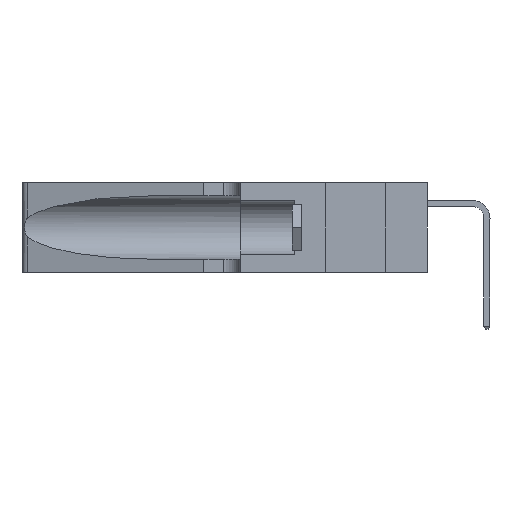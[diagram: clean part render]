
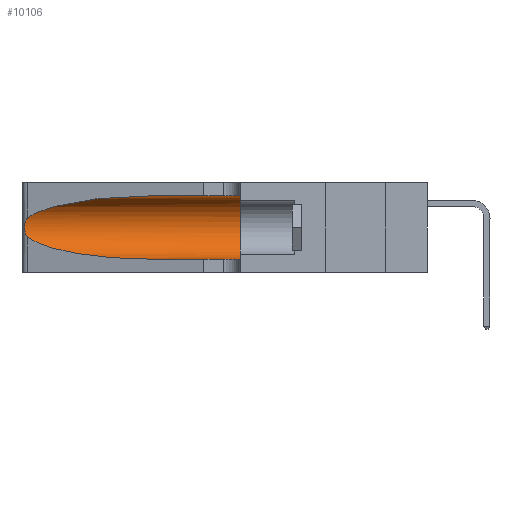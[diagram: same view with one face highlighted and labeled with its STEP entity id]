
A CAD part, left-side view. The second image highlights one B-rep face of the part: STEP entity #10106.
In plain terms, the highlighted cylindrical face has radius 3.308 mm (diameter 6.617 mm), a partial arc.
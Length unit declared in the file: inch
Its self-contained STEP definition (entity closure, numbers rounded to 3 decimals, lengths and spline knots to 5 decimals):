
#382 = ORIENTED_EDGE ( 'NONE', *, *, #32515, .T. ) ;
#560 = VERTEX_POINT ( 'NONE', #32320 ) ;
#607 = LINE ( 'NONE', #25444, #25450 ) ;
#755 = CARTESIAN_POINT ( 'NONE',  ( 0.25789, 1.23486, 0.15765 ) ) ;
#821 = EDGE_LOOP ( 'NONE', ( #34438, #382, #29075, #11281, #27365, #1887 ) ) ;
#831 = CARTESIAN_POINT ( 'NONE',  ( 0.1305, 0.72297, 0.31525 ) ) ;
#1108 = EDGE_CURVE ( 'NONE', #21197, #4653, #32869, .T. ) ;
#1227 = CYLINDRICAL_SURFACE ( 'NONE', #13392, 0.13025 ) ;
#1328 = CARTESIAN_POINT ( 'NONE',  ( 0.18966, 0.96281, 0.05475 ) ) ;
#1887 = ORIENTED_EDGE ( 'NONE', *, *, #24111, .F. ) ;
#3818 = CARTESIAN_POINT ( 'NONE',  ( 0.25555, 1.22993, 0.14849 ) ) ;
#4381 = CARTESIAN_POINT ( 'NONE',  ( 0.1305, 0.72297, 0.05475 ) ) ;
#4653 = VERTEX_POINT ( 'NONE', #5918 ) ;
#5918 = CARTESIAN_POINT ( 'NONE',  ( 0.25487, 1.22718, 0.22369 ) ) ;
#7617 = DIRECTION ( 'NONE',  ( 0., -1., 0. ) ) ;
#7729 = VERTEX_POINT ( 'NONE', #23437 ) ;
#8847 = DIRECTION ( 'NONE',  ( 0., 1., 0. ) ) ;
#9166 = DIRECTION ( 'NONE',  ( 0., 0., -1. ) ) ;
#9747 = CARTESIAN_POINT ( 'NONE',  ( 0.25787, 1.23484, 0.2124 ) ) ;
#10106 = ADVANCED_FACE ( 'NONE', ( #11139 ), #1227, .F. ) ;
#10968 = DIRECTION ( 'NONE',  ( 0., -1., 0. ) ) ;
#11139 = FACE_OUTER_BOUND ( 'NONE', #821, .T. ) ;
#11168 = EDGE_CURVE ( 'NONE', #7729, #560, #19124, .T. ) ;
#11281 = ORIENTED_EDGE ( 'NONE', *, *, #17929, .T. ) ;
#11406 = CARTESIAN_POINT ( 'NONE',  ( 0.2373, 1.15595, 0.28018 ) ) ;
#12757 = CARTESIAN_POINT ( 'NONE',  ( 0.26018, 1.23835, 0.19895 ) ) ;
#13392 = AXIS2_PLACEMENT_3D ( 'NONE', #29950, #35878, #9166 ) ;
#15641 = CARTESIAN_POINT ( 'NONE',  ( 0.25487, 1.22718, 0.22369 ) ) ;
#15776 = CARTESIAN_POINT ( 'NONE',  ( 0.26075, 1.23896, 0.178 ) ) ;
#15816 = B_SPLINE_CURVE_WITH_KNOTS ( 'NONE', 3,
 ( #15641, #24593, #27563, #9747, #30521, #12757, #33471, #15776, #36446, #18766, #755, #21733, #3818, #24718 ),
 .UNSPECIFIED., .F., .F.,
 ( 4, 2, 2, 2, 2, 2, 4 ),
 ( 0., 0.00027, 0.00053, 0.00107, 0.0016, 0.00187, 0.00214 ),
 .UNSPECIFIED. ) ;
#16170 = VECTOR ( 'NONE', #10968, 39.37008 ) ;
#17423 = CARTESIAN_POINT ( 'NONE',  ( 0.1305, 0.72297, 0.31525 ) ) ;
#17929 = EDGE_CURVE ( 'NONE', #29703, #560, #607, .T. ) ;
#18766 = CARTESIAN_POINT ( 'NONE',  ( 0.25856, 1.23593, 0.16098 ) ) ;
#19124 = CIRCLE ( 'NONE', #19183, 0.13025 ) ;
#19183 = AXIS2_PLACEMENT_3D ( 'NONE', #26673, #8847, #29626 ) ;
#19988 = EDGE_CURVE ( 'NONE', #35842, #29703, #38396, .T. ) ;
#20405 = CARTESIAN_POINT ( 'NONE',  ( 0.25487, 1.22718, 0.22369 ) ) ;
#21197 = VERTEX_POINT ( 'NONE', #831 ) ;
#21733 = CARTESIAN_POINT ( 'NONE',  ( 0.25639, 1.23186, 0.15144 ) ) ;
#23437 = CARTESIAN_POINT ( 'NONE',  ( 0.1305, 0.35, 0.31525 ) ) ;
#24111 = EDGE_CURVE ( 'NONE', #21197, #7729, #31914, .T. ) ;
#24455 = CARTESIAN_POINT ( 'NONE',  ( 0.1305, 0.72297, 0.05475 ) ) ;
#24593 = CARTESIAN_POINT ( 'NONE',  ( 0.25555, 1.22994, 0.2215 ) ) ;
#24718 = CARTESIAN_POINT ( 'NONE',  ( 0.25487, 1.22718, 0.14631 ) ) ;
#25444 = CARTESIAN_POINT ( 'NONE',  ( 0.1305, 1.61858, 0.05475 ) ) ;
#25450 = VECTOR ( 'NONE', #7617, 39.37008 ) ;
#25818 = CARTESIAN_POINT ( 'NONE',  ( 0.1305, 1.61858, 0.31525 ) ) ;
#26673 = CARTESIAN_POINT ( 'NONE',  ( 0.1305, 0.35, 0.185 ) ) ;
#27365 = ORIENTED_EDGE ( 'NONE', *, *, #11168, .F. ) ;
#27563 = CARTESIAN_POINT ( 'NONE',  ( 0.25639, 1.23184, 0.21858 ) ) ;
#29075 = ORIENTED_EDGE ( 'NONE', *, *, #19988, .T. ) ;
#29626 = DIRECTION ( 'NONE',  ( 0., 0., 1. ) ) ;
#29703 = VERTEX_POINT ( 'NONE', #24455 ) ;
#29950 = CARTESIAN_POINT ( 'NONE',  ( 0.1305, 1.61858, 0.185 ) ) ;
#30521 = CARTESIAN_POINT ( 'NONE',  ( 0.25854, 1.2359, 0.20912 ) ) ;
#31059 = CARTESIAN_POINT ( 'NONE',  ( 0.25487, 1.22718, 0.14631 ) ) ;
#31914 = LINE ( 'NONE', #25818, #16170 ) ;
#32148 = CARTESIAN_POINT ( 'NONE',  ( 0.18966, 0.96281, 0.31525 ) ) ;
#32320 = CARTESIAN_POINT ( 'NONE',  ( 0.1305, 0.35, 0.05475 ) ) ;
#32515 = EDGE_CURVE ( 'NONE', #4653, #35842, #15816, .T. ) ;
#32869 =( BOUNDED_CURVE ( )  B_SPLINE_CURVE ( 3, ( #17423, #32148, #11406, #20405 ),
 .UNSPECIFIED., .F., .T. ) 
 B_SPLINE_CURVE_WITH_KNOTS ( ( 4, 4 ),
 ( 1.5708, 2.84003 ),
 .UNSPECIFIED. ) 
 CURVE ( )  GEOMETRIC_REPRESENTATION_ITEM ( )  RATIONAL_B_SPLINE_CURVE ( ( 1., 0.87, 0.87, 1. ) ) 
 REPRESENTATION_ITEM ( '' )  );
#33471 = CARTESIAN_POINT ( 'NONE',  ( 0.26075, 1.23896, 0.19203 ) ) ;
#34438 = ORIENTED_EDGE ( 'NONE', *, *, #1108, .T. ) ;
#35842 = VERTEX_POINT ( 'NONE', #38477 ) ;
#35878 = DIRECTION ( 'NONE',  ( 0., -1., 0. ) ) ;
#36446 = CARTESIAN_POINT ( 'NONE',  ( 0.26017, 1.23833, 0.17102 ) ) ;
#36991 = CARTESIAN_POINT ( 'NONE',  ( 0.2373, 1.15595, 0.08982 ) ) ;
#38396 =( BOUNDED_CURVE ( )  B_SPLINE_CURVE ( 3, ( #31059, #36991, #1328, #4381 ),
 .UNSPECIFIED., .F., .F. ) 
 B_SPLINE_CURVE_WITH_KNOTS ( ( 4, 4 ),
 ( 3.44316, 4.71239 ),
 .UNSPECIFIED. ) 
 CURVE ( )  GEOMETRIC_REPRESENTATION_ITEM ( )  RATIONAL_B_SPLINE_CURVE ( ( 1., 0.87, 0.87, 1. ) ) 
 REPRESENTATION_ITEM ( '' )  );
#38477 = CARTESIAN_POINT ( 'NONE',  ( 0.25487, 1.22718, 0.14631 ) ) ;
